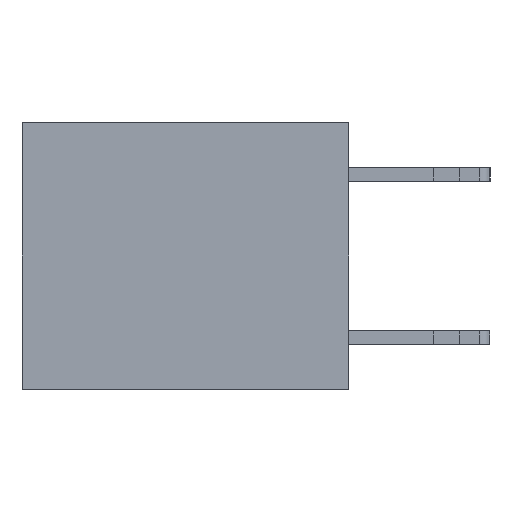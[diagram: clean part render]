
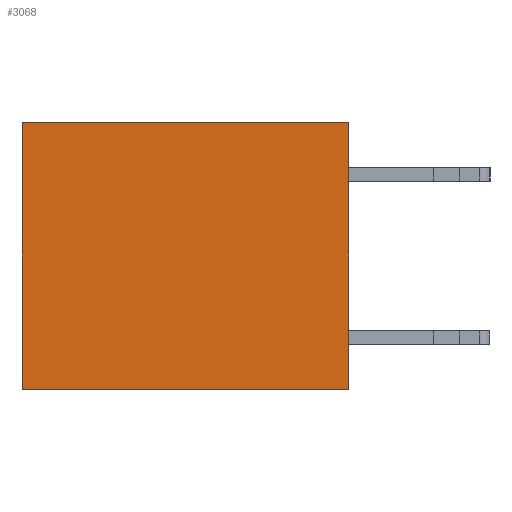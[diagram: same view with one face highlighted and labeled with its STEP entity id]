
A CAD part, left-side view. The second image highlights one B-rep face of the part: STEP entity #3068.
In plain terms, the highlighted planar face has unit normal (-1, 0, 0).
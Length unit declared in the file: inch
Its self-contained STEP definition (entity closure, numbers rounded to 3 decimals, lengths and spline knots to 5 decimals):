
#520 = LINE ( 'NONE', #3784, #11982 ) ;
#594 = VERTEX_POINT ( 'NONE', #7575 ) ;
#1074 = EDGE_CURVE ( 'NONE', #16841, #15285, #520, .T. ) ;
#1393 = ORIENTED_EDGE ( 'NONE', *, *, #12642, .T. ) ;
#1500 = CARTESIAN_POINT ( 'NONE',  ( 0.3165, 0., -0.49 ) ) ;
#1622 = VECTOR ( 'NONE', #14900, 39.37008 ) ;
#2008 = LINE ( 'NONE', #7096, #3003 ) ;
#2121 = DIRECTION ( 'NONE',  ( 1., 0., 0. ) ) ;
#3003 = VECTOR ( 'NONE', #7155, 39.37008 ) ;
#3068 = ADVANCED_FACE ( 'NONE', ( #16593 ), #7329, .F. ) ;
#3784 = CARTESIAN_POINT ( 'NONE',  ( 0.3165, 0., -0.49 ) ) ;
#4745 = DIRECTION ( 'NONE',  ( 0., 0., -1. ) ) ;
#4905 = VECTOR ( 'NONE', #10668, 39.37008 ) ;
#5415 = DIRECTION ( 'NONE',  ( 0., 0., -1. ) ) ;
#6283 = EDGE_CURVE ( 'NONE', #594, #8710, #2008, .T. ) ;
#7024 = CARTESIAN_POINT ( 'NONE',  ( 0.3165, 0., 0. ) ) ;
#7096 = CARTESIAN_POINT ( 'NONE',  ( 0.3165, 0.6, -0.49 ) ) ;
#7155 = DIRECTION ( 'NONE',  ( 0., 0., -1. ) ) ;
#7329 = PLANE ( 'NONE',  #15331 ) ;
#7575 = CARTESIAN_POINT ( 'NONE',  ( 0.3165, 0.6, 0. ) ) ;
#8381 = LINE ( 'NONE', #1500, #4905 ) ;
#8710 = VERTEX_POINT ( 'NONE', #9666 ) ;
#9408 = LINE ( 'NONE', #7024, #1622 ) ;
#9666 = CARTESIAN_POINT ( 'NONE',  ( 0.3165, 0.6, -0.49 ) ) ;
#9754 = EDGE_LOOP ( 'NONE', ( #10417, #11235, #11573, #1393 ) ) ;
#9965 = CARTESIAN_POINT ( 'NONE',  ( 0.3165, 0., -0.49 ) ) ;
#10417 = ORIENTED_EDGE ( 'NONE', *, *, #6283, .T. ) ;
#10668 = DIRECTION ( 'NONE',  ( 0., 1., 0. ) ) ;
#11182 = CARTESIAN_POINT ( 'NONE',  ( 0.3165, 0., -0.49 ) ) ;
#11235 = ORIENTED_EDGE ( 'NONE', *, *, #15061, .F. ) ;
#11573 = ORIENTED_EDGE ( 'NONE', *, *, #1074, .F. ) ;
#11982 = VECTOR ( 'NONE', #5415, 39.37008 ) ;
#12642 = EDGE_CURVE ( 'NONE', #16841, #594, #9408, .T. ) ;
#14900 = DIRECTION ( 'NONE',  ( 0., 1., 0. ) ) ;
#15061 = EDGE_CURVE ( 'NONE', #15285, #8710, #8381, .T. ) ;
#15285 = VERTEX_POINT ( 'NONE', #11182 ) ;
#15316 = CARTESIAN_POINT ( 'NONE',  ( 0.3165, 0., 0. ) ) ;
#15331 = AXIS2_PLACEMENT_3D ( 'NONE', #9965, #2121, #4745 ) ;
#16593 = FACE_OUTER_BOUND ( 'NONE', #9754, .T. ) ;
#16841 = VERTEX_POINT ( 'NONE', #15316 ) ;
